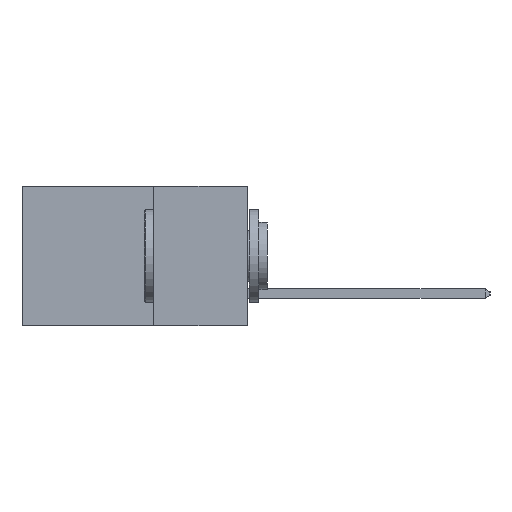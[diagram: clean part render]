
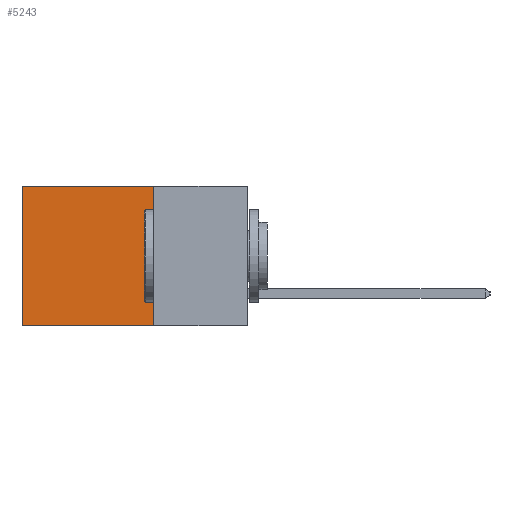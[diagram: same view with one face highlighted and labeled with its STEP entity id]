
A CAD part, left-side view. The second image highlights one B-rep face of the part: STEP entity #5243.
In plain terms, the highlighted planar face has unit normal (-1, 0, 0).
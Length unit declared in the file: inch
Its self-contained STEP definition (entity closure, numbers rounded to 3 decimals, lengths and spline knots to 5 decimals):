
#134 = CARTESIAN_POINT ( 'NONE',  ( 0.298, 0.25, -0.37 ) ) ;
#340 = CARTESIAN_POINT ( 'NONE',  ( 0.298, 0.6, 0. ) ) ;
#597 = EDGE_CURVE ( 'NONE', #12959, #21432, #12016, .T. ) ;
#1189 = PLANE ( 'NONE',  #17465 ) ;
#1731 = EDGE_CURVE ( 'NONE', #21432, #6897, #6792, .T. ) ;
#2165 = VECTOR ( 'NONE', #11570, 39.37008 ) ;
#2791 = VECTOR ( 'NONE', #5130, 39.37008 ) ;
#3005 = CARTESIAN_POINT ( 'NONE',  ( 0.298, 0.25, 0. ) ) ;
#3334 = FACE_OUTER_BOUND ( 'NONE', #19609, .T. ) ;
#3545 = VECTOR ( 'NONE', #9183, 39.37008 ) ;
#4974 = CARTESIAN_POINT ( 'NONE',  ( 0.298, 0.25, 0. ) ) ;
#5130 = DIRECTION ( 'NONE',  ( 0., 1., 0. ) ) ;
#5243 = ADVANCED_FACE ( 'NONE', ( #3334 ), #1189, .F. ) ;
#5623 = CARTESIAN_POINT ( 'NONE',  ( 0.298, 0.25, 0. ) ) ;
#6198 = DIRECTION ( 'NONE',  ( 0., 0., -1. ) ) ;
#6341 = DIRECTION ( 'NONE',  ( 1., 0., 0. ) ) ;
#6792 = LINE ( 'NONE', #13579, #2165 ) ;
#6897 = VERTEX_POINT ( 'NONE', #9025 ) ;
#6956 = EDGE_CURVE ( 'NONE', #8127, #6897, #17196, .T. ) ;
#6969 = ORIENTED_EDGE ( 'NONE', *, *, #1731, .T. ) ;
#7378 = LINE ( 'NONE', #15771, #15427 ) ;
#7420 = CARTESIAN_POINT ( 'NONE',  ( 0.298, 0.25, -0.37 ) ) ;
#8127 = VERTEX_POINT ( 'NONE', #134 ) ;
#9025 = CARTESIAN_POINT ( 'NONE',  ( 0.298, 0.6, -0.37 ) ) ;
#9183 = DIRECTION ( 'NONE',  ( 0., 1., 0. ) ) ;
#9463 = EDGE_CURVE ( 'NONE', #12959, #8127, #7378, .T. ) ;
#11570 = DIRECTION ( 'NONE',  ( 0., 0., -1. ) ) ;
#12016 = LINE ( 'NONE', #4974, #2791 ) ;
#12443 = DIRECTION ( 'NONE',  ( 0., 0., -1. ) ) ;
#12959 = VERTEX_POINT ( 'NONE', #3005 ) ;
#13579 = CARTESIAN_POINT ( 'NONE',  ( 0.298, 0.6, 0. ) ) ;
#14066 = ORIENTED_EDGE ( 'NONE', *, *, #597, .T. ) ;
#15427 = VECTOR ( 'NONE', #12443, 39.37008 ) ;
#15771 = CARTESIAN_POINT ( 'NONE',  ( 0.298, 0.25, 0. ) ) ;
#16528 = ORIENTED_EDGE ( 'NONE', *, *, #9463, .F. ) ;
#17196 = LINE ( 'NONE', #7420, #3545 ) ;
#17465 = AXIS2_PLACEMENT_3D ( 'NONE', #5623, #6341, #6198 ) ;
#19609 = EDGE_LOOP ( 'NONE', ( #6969, #21042, #16528, #14066 ) ) ;
#21042 = ORIENTED_EDGE ( 'NONE', *, *, #6956, .F. ) ;
#21432 = VERTEX_POINT ( 'NONE', #340 ) ;
